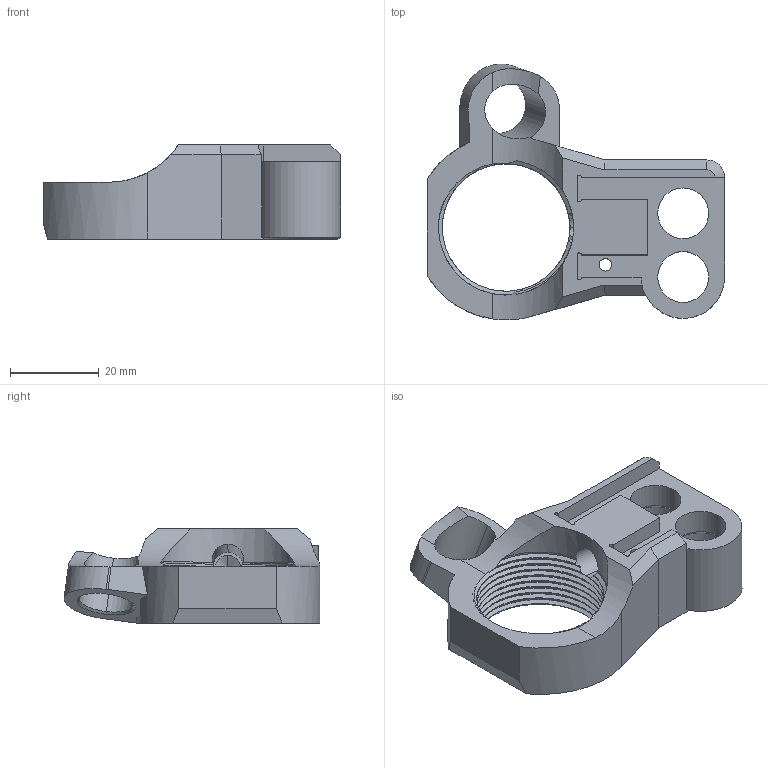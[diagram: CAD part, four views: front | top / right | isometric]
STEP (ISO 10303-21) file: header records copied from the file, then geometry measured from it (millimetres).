
FILE_DESCRIPTION (( 'STEP AP203' ), '1' );
FILE_NAME ('AF-HF-LR-PRT-002-STEP_NO_SUPPORTS.STEP', '2020-10-09T03:35:41', ( '' ), ( '' ), 'SwSTEP 2.0', 'SolidWorks 2018', '' );
FILE_SCHEMA (( 'CONFIG_CONTROL_DESIGN' ));
Length unit declared in the file: inch
Products named in the file (1): AF-HF-LR-PRT-002-STEP_NO_SUPPORTS
Bounding box: 66.83 x 57.55 x 21.17 mm (x, y, z)
Volume: 23810.7 mm3; surface area: 11645.7 mm2
Topology: 1 solids, 1 shells, 119 faces, 332 edges, 211 vertices
Faces by surface type: cylinder 54, plane 33, cone 21, bspline 11
Entity records: 7829 total; most frequent: CARTESIAN_POINT 4970, ORIENTED_EDGE 656, DIRECTION 510, EDGE_CURVE 328, VERTEX_POINT 211, AXIS2_PLACEMENT_3D 188, LINE 134, VECTOR 134
